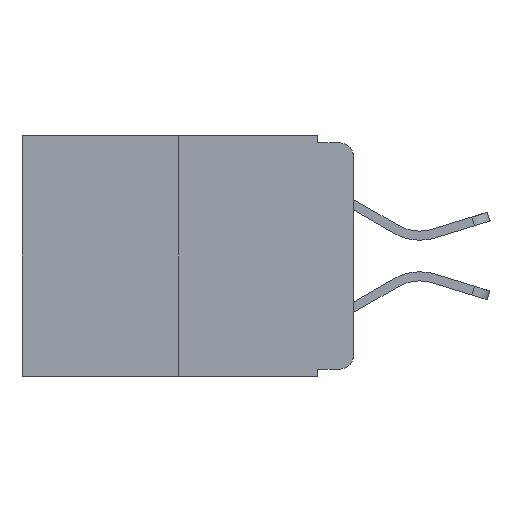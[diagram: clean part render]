
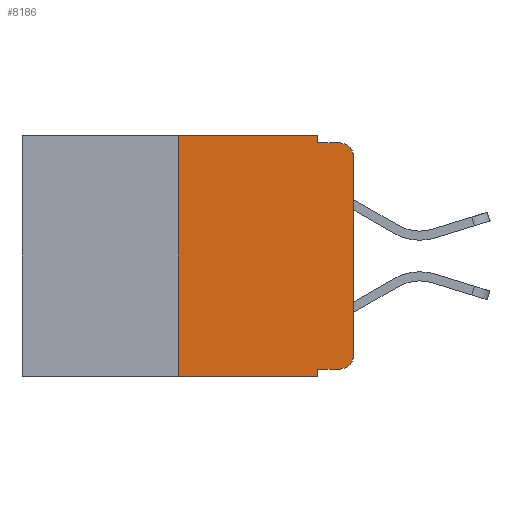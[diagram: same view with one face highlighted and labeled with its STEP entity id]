
A CAD part, left-side view. The second image highlights one B-rep face of the part: STEP entity #8186.
In plain terms, the highlighted planar face has unit normal (-1, 0, 0).
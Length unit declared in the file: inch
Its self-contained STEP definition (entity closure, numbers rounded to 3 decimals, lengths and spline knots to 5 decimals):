
#10 = ORIENTED_EDGE ( 'NONE', *, *, #3639, .F. ) ;
#51 = ORIENTED_EDGE ( 'NONE', *, *, #1410, .T. ) ;
#428 = CARTESIAN_POINT ( 'NONE',  ( 0., 0.25, 0. ) ) ;
#443 = VECTOR ( 'NONE', #9552, 39.37008 ) ;
#688 = EDGE_CURVE ( 'NONE', #5315, #1271, #7045, .T. ) ;
#810 = VERTEX_POINT ( 'NONE', #4982 ) ;
#864 = LINE ( 'NONE', #8942, #8451 ) ;
#885 = AXIS2_PLACEMENT_3D ( 'NONE', #4374, #10054, #5249 ) ;
#1271 = VERTEX_POINT ( 'NONE', #3085 ) ;
#1410 = EDGE_CURVE ( 'NONE', #1271, #3812, #11340, .T. ) ;
#1786 = DIRECTION ( 'NONE',  ( 0., -1., 0. ) ) ;
#1951 = ORIENTED_EDGE ( 'NONE', *, *, #5960, .T. ) ;
#2042 = DIRECTION ( 'NONE',  ( 0., 0., 1. ) ) ;
#2092 = ORIENTED_EDGE ( 'NONE', *, *, #688, .T. ) ;
#2174 = EDGE_CURVE ( 'NONE', #6052, #4613, #4654, .T. ) ;
#2279 = ORIENTED_EDGE ( 'NONE', *, *, #2174, .F. ) ;
#2299 = ORIENTED_EDGE ( 'NONE', *, *, #7390, .T. ) ;
#2358 = ORIENTED_EDGE ( 'NONE', *, *, #2919, .F. ) ;
#2498 = ORIENTED_EDGE ( 'NONE', *, *, #4836, .T. ) ;
#2544 = ORIENTED_EDGE ( 'NONE', *, *, #4242, .F. ) ;
#2608 = CARTESIAN_POINT ( 'NONE',  ( 0., 0.051, -0.01 ) ) ;
#2830 = ORIENTED_EDGE ( 'NONE', *, *, #9264, .F. ) ;
#2919 = EDGE_CURVE ( 'NONE', #5315, #810, #10553, .T. ) ;
#3085 = CARTESIAN_POINT ( 'NONE',  ( 0., 0.02, -0.333 ) ) ;
#3088 = CARTESIAN_POINT ( 'NONE',  ( 0., 0.051, -0.01 ) ) ;
#3535 = CARTESIAN_POINT ( 'NONE',  ( 0., 0.25, -0.343 ) ) ;
#3639 = EDGE_CURVE ( 'NONE', #3873, #6345, #9571, .T. ) ;
#3684 = DIRECTION ( 'NONE',  ( 0., 0., -1. ) ) ;
#3802 = CARTESIAN_POINT ( 'NONE',  ( 0., 0.473, 0. ) ) ;
#3812 = VERTEX_POINT ( 'NONE', #3963 ) ;
#3864 = VECTOR ( 'NONE', #1786, 39.37008 ) ;
#3873 = VERTEX_POINT ( 'NONE', #3088 ) ;
#3884 = AXIS2_PLACEMENT_3D ( 'NONE', #5477, #11047, #6312 ) ;
#3963 = CARTESIAN_POINT ( 'NONE',  ( 0., 0., -0.313 ) ) ;
#4242 = EDGE_CURVE ( 'NONE', #9027, #3873, #9316, .T. ) ;
#4374 = CARTESIAN_POINT ( 'NONE',  ( 0., 0.02, -0.03 ) ) ;
#4426 = EDGE_LOOP ( 'NONE', ( #2498, #1951, #10, #2544, #2830, #2279, #2299, #2358, #2092, #51 ) ) ;
#4545 = DIRECTION ( 'NONE',  ( 0., -1., 0. ) ) ;
#4613 = VERTEX_POINT ( 'NONE', #4708 ) ;
#4654 = LINE ( 'NONE', #428, #8739 ) ;
#4679 = CARTESIAN_POINT ( 'NONE',  ( 0., 0.02, -0.01 ) ) ;
#4708 = CARTESIAN_POINT ( 'NONE',  ( 0., 0.25, 0. ) ) ;
#4836 = EDGE_CURVE ( 'NONE', #3812, #6778, #864, .T. ) ;
#4982 = CARTESIAN_POINT ( 'NONE',  ( 0., 0.051, -0.343 ) ) ;
#5249 = DIRECTION ( 'NONE',  ( 0., 0., -1. ) ) ;
#5278 = VECTOR ( 'NONE', #10880, 39.37008 ) ;
#5315 = VERTEX_POINT ( 'NONE', #8725 ) ;
#5477 = CARTESIAN_POINT ( 'NONE',  ( 0., 0.473, 0. ) ) ;
#5648 = CIRCLE ( 'NONE', #885, 0.02 ) ;
#5960 = EDGE_CURVE ( 'NONE', #6778, #6345, #5648, .T. ) ;
#6052 = VERTEX_POINT ( 'NONE', #3535 ) ;
#6162 = CARTESIAN_POINT ( 'NONE',  ( 0., 0.051, 0. ) ) ;
#6312 = DIRECTION ( 'NONE',  ( 0., 0., -1. ) ) ;
#6326 = VECTOR ( 'NONE', #9947, 39.37008 ) ;
#6345 = VERTEX_POINT ( 'NONE', #4679 ) ;
#6778 = VERTEX_POINT ( 'NONE', #7572 ) ;
#7045 = LINE ( 'NONE', #9337, #11000 ) ;
#7085 = DIRECTION ( 'NONE',  ( 0., -1., 0. ) ) ;
#7390 = EDGE_CURVE ( 'NONE', #6052, #810, #8539, .T. ) ;
#7468 = VECTOR ( 'NONE', #7085, 39.37008 ) ;
#7572 = CARTESIAN_POINT ( 'NONE',  ( 0., 0., -0.03 ) ) ;
#8113 = DIRECTION ( 'NONE',  ( 0., 0., 1. ) ) ;
#8186 = ADVANCED_FACE ( 'NONE', ( #10973 ), #10277, .F. ) ;
#8451 = VECTOR ( 'NONE', #8113, 39.37008 ) ;
#8539 = LINE ( 'NONE', #11193, #3864 ) ;
#8725 = CARTESIAN_POINT ( 'NONE',  ( 0., 0.051, -0.333 ) ) ;
#8739 = VECTOR ( 'NONE', #2042, 39.37008 ) ;
#8942 = CARTESIAN_POINT ( 'NONE',  ( 0., 0., 0. ) ) ;
#9027 = VERTEX_POINT ( 'NONE', #6162 ) ;
#9158 = CARTESIAN_POINT ( 'NONE',  ( 0., 0.051, 0. ) ) ;
#9264 = EDGE_CURVE ( 'NONE', #4613, #9027, #9746, .T. ) ;
#9316 = LINE ( 'NONE', #10913, #5278 ) ;
#9337 = CARTESIAN_POINT ( 'NONE',  ( 0., 0.051, -0.333 ) ) ;
#9552 = DIRECTION ( 'NONE',  ( 0., -1., 0. ) ) ;
#9571 = LINE ( 'NONE', #2608, #7468 ) ;
#9746 = LINE ( 'NONE', #3802, #443 ) ;
#9947 = DIRECTION ( 'NONE',  ( 0., 0., -1. ) ) ;
#10054 = DIRECTION ( 'NONE',  ( -1., 0., 0. ) ) ;
#10277 = PLANE ( 'NONE',  #3884 ) ;
#10464 = AXIS2_PLACEMENT_3D ( 'NONE', #11044, #11048, #3684 ) ;
#10553 = LINE ( 'NONE', #9158, #6326 ) ;
#10880 = DIRECTION ( 'NONE',  ( 0., 0., -1. ) ) ;
#10913 = CARTESIAN_POINT ( 'NONE',  ( 0., 0.051, 0. ) ) ;
#10973 = FACE_OUTER_BOUND ( 'NONE', #4426, .T. ) ;
#11000 = VECTOR ( 'NONE', #4545, 39.37008 ) ;
#11044 = CARTESIAN_POINT ( 'NONE',  ( 0., 0.02, -0.313 ) ) ;
#11047 = DIRECTION ( 'NONE',  ( 1., 0., 0. ) ) ;
#11048 = DIRECTION ( 'NONE',  ( -1., 0., 0. ) ) ;
#11193 = CARTESIAN_POINT ( 'NONE',  ( 0., 0.473, -0.343 ) ) ;
#11340 = CIRCLE ( 'NONE', #10464, 0.02 ) ;
